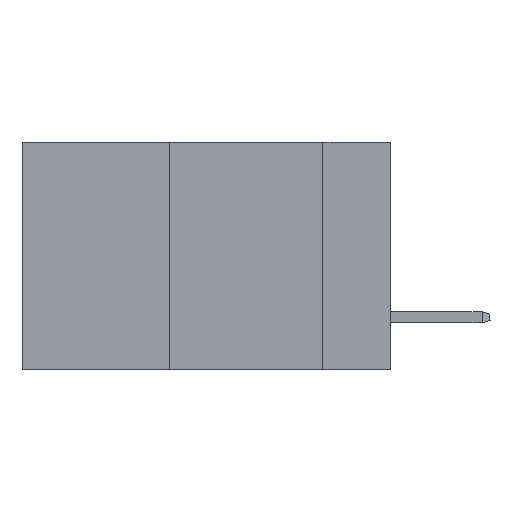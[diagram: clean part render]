
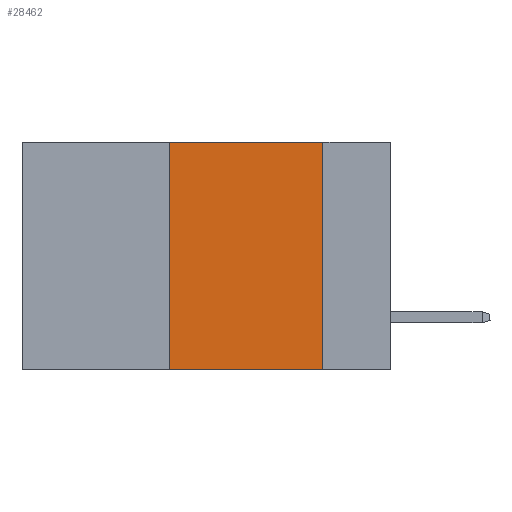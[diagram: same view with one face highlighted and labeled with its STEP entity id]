
A CAD part, left-side view. The second image highlights one B-rep face of the part: STEP entity #28462.
In plain terms, the highlighted planar face has unit normal (-1, 0, 0).
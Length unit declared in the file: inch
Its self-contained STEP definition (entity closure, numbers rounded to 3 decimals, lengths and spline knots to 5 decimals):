
#810 = CARTESIAN_POINT ( 'NONE',  ( 0., 0.11, 0. ) ) ;
#942 = CARTESIAN_POINT ( 'NONE',  ( 0., 0.6, 0. ) ) ;
#2073 = EDGE_CURVE ( 'NONE', #9149, #29413, #15940, .T. ) ;
#3743 = ORIENTED_EDGE ( 'NONE', *, *, #34671, .F. ) ;
#4243 = LINE ( 'NONE', #9730, #10619 ) ;
#8101 = DIRECTION ( 'NONE',  ( 0., 0., -1. ) ) ;
#8231 = CARTESIAN_POINT ( 'NONE',  ( 0., 0.11, 0. ) ) ;
#8509 = AXIS2_PLACEMENT_3D ( 'NONE', #23556, #12370, #29358 ) ;
#9149 = VERTEX_POINT ( 'NONE', #27559 ) ;
#9225 = PLANE ( 'NONE',  #8509 ) ;
#9730 = CARTESIAN_POINT ( 'NONE',  ( 0., 0.6, -0.37 ) ) ;
#10619 = VECTOR ( 'NONE', #29881, 39.37008 ) ;
#11968 = FACE_OUTER_BOUND ( 'NONE', #30067, .T. ) ;
#12370 = DIRECTION ( 'NONE',  ( 1., 0., 0. ) ) ;
#14034 = EDGE_CURVE ( 'NONE', #29413, #34060, #21741, .T. ) ;
#14774 = LINE ( 'NONE', #8231, #20632 ) ;
#15783 = CARTESIAN_POINT ( 'NONE',  ( 0., 0.36, 0. ) ) ;
#15940 = LINE ( 'NONE', #15783, #35810 ) ;
#20374 = VECTOR ( 'NONE', #20766, 39.37008 ) ;
#20632 = VECTOR ( 'NONE', #8101, 39.37008 ) ;
#20766 = DIRECTION ( 'NONE',  ( 0., -1., 0. ) ) ;
#21741 = LINE ( 'NONE', #942, #20374 ) ;
#23556 = CARTESIAN_POINT ( 'NONE',  ( 0., 0.6, 0. ) ) ;
#26762 = CARTESIAN_POINT ( 'NONE',  ( 0., 0.36, 0. ) ) ;
#27559 = CARTESIAN_POINT ( 'NONE',  ( 0., 0.36, -0.37 ) ) ;
#28462 = ADVANCED_FACE ( 'NONE', ( #11968 ), #9225, .F. ) ;
#29358 = DIRECTION ( 'NONE',  ( 0., 0., -1. ) ) ;
#29413 = VERTEX_POINT ( 'NONE', #26762 ) ;
#29881 = DIRECTION ( 'NONE',  ( 0., -1., 0. ) ) ;
#30067 = EDGE_LOOP ( 'NONE', ( #3743, #31212, #36486, #35982 ) ) ;
#30402 = DIRECTION ( 'NONE',  ( 0., 0., 1. ) ) ;
#31052 = VERTEX_POINT ( 'NONE', #37202 ) ;
#31212 = ORIENTED_EDGE ( 'NONE', *, *, #14034, .F. ) ;
#31683 = EDGE_CURVE ( 'NONE', #9149, #31052, #4243, .T. ) ;
#34060 = VERTEX_POINT ( 'NONE', #810 ) ;
#34671 = EDGE_CURVE ( 'NONE', #34060, #31052, #14774, .T. ) ;
#35810 = VECTOR ( 'NONE', #30402, 39.37008 ) ;
#35982 = ORIENTED_EDGE ( 'NONE', *, *, #31683, .T. ) ;
#36486 = ORIENTED_EDGE ( 'NONE', *, *, #2073, .F. ) ;
#37202 = CARTESIAN_POINT ( 'NONE',  ( 0., 0.11, -0.37 ) ) ;
